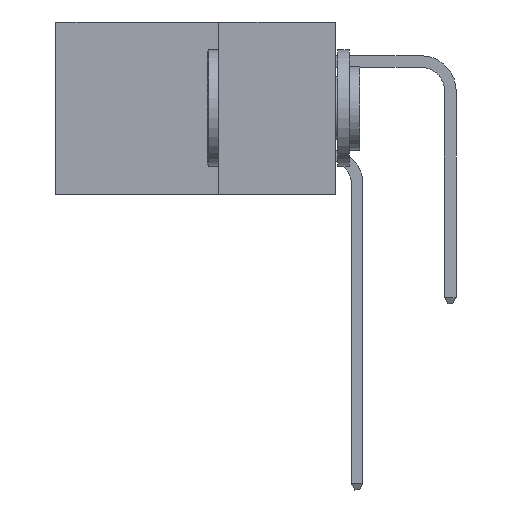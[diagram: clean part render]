
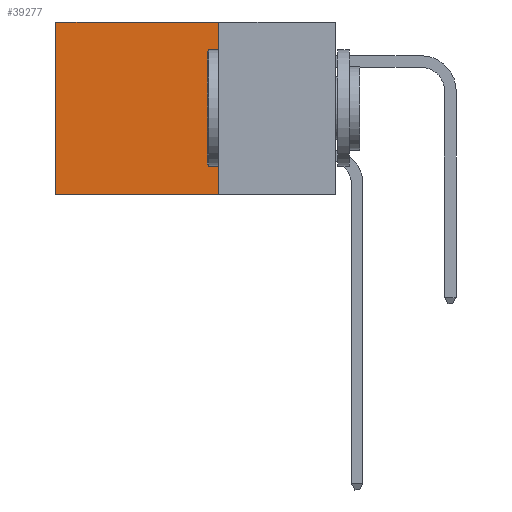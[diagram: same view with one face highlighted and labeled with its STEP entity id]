
A CAD part, left-side view. The second image highlights one B-rep face of the part: STEP entity #39277.
In plain terms, the highlighted planar face has unit normal (-1, 0, 0).
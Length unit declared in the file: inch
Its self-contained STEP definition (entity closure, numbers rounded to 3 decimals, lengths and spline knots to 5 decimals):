
#844 = VERTEX_POINT ( 'NONE', #34008 ) ;
#2474 = LINE ( 'NONE', #29731, #31496 ) ;
#5614 = VECTOR ( 'NONE', #31732, 39.37008 ) ;
#6262 = DIRECTION ( 'NONE',  ( 0., 0., -1. ) ) ;
#7840 = VECTOR ( 'NONE', #37528, 39.37008 ) ;
#9372 = DIRECTION ( 'NONE',  ( 0., 0., -1. ) ) ;
#11034 = VERTEX_POINT ( 'NONE', #16763 ) ;
#11585 = EDGE_CURVE ( 'NONE', #22320, #32104, #30597, .T. ) ;
#12231 = CARTESIAN_POINT ( 'NONE',  ( 0.2875, 0.25, -0.37 ) ) ;
#15916 = ORIENTED_EDGE ( 'NONE', *, *, #34098, .T. ) ;
#16762 = DIRECTION ( 'NONE',  ( 1., 0., 0. ) ) ;
#16763 = CARTESIAN_POINT ( 'NONE',  ( 0.2875, 0.25, 0. ) ) ;
#18892 = CARTESIAN_POINT ( 'NONE',  ( 0.2875, 0.25, -0.37 ) ) ;
#20705 = CARTESIAN_POINT ( 'NONE',  ( 0.2875, 0.25, 0. ) ) ;
#21686 = VECTOR ( 'NONE', #22266, 39.37008 ) ;
#22266 = DIRECTION ( 'NONE',  ( 0., 1., 0. ) ) ;
#22320 = VERTEX_POINT ( 'NONE', #12231 ) ;
#25436 = AXIS2_PLACEMENT_3D ( 'NONE', #36960, #16762, #6262 ) ;
#26860 = EDGE_CURVE ( 'NONE', #11034, #22320, #30504, .T. ) ;
#28300 = LINE ( 'NONE', #28796, #5614 ) ;
#28796 = CARTESIAN_POINT ( 'NONE',  ( 0.2875, 0.25, 0. ) ) ;
#29137 = FACE_OUTER_BOUND ( 'NONE', #35464, .T. ) ;
#29329 = ORIENTED_EDGE ( 'NONE', *, *, #26860, .F. ) ;
#29731 = CARTESIAN_POINT ( 'NONE',  ( 0.2875, 0.6, 0. ) ) ;
#30290 = ORIENTED_EDGE ( 'NONE', *, *, #34430, .T. ) ;
#30504 = LINE ( 'NONE', #20705, #7840 ) ;
#30597 = LINE ( 'NONE', #18892, #21686 ) ;
#31496 = VECTOR ( 'NONE', #9372, 39.37008 ) ;
#31732 = DIRECTION ( 'NONE',  ( 0., 1., 0. ) ) ;
#32104 = VERTEX_POINT ( 'NONE', #32429 ) ;
#32429 = CARTESIAN_POINT ( 'NONE',  ( 0.2875, 0.6, -0.37 ) ) ;
#33808 = PLANE ( 'NONE',  #25436 ) ;
#34008 = CARTESIAN_POINT ( 'NONE',  ( 0.2875, 0.6, 0. ) ) ;
#34098 = EDGE_CURVE ( 'NONE', #844, #32104, #2474, .T. ) ;
#34430 = EDGE_CURVE ( 'NONE', #11034, #844, #28300, .T. ) ;
#35464 = EDGE_LOOP ( 'NONE', ( #15916, #37296, #29329, #30290 ) ) ;
#36960 = CARTESIAN_POINT ( 'NONE',  ( 0.2875, 0.25, 0. ) ) ;
#37296 = ORIENTED_EDGE ( 'NONE', *, *, #11585, .F. ) ;
#37528 = DIRECTION ( 'NONE',  ( 0., 0., -1. ) ) ;
#39277 = ADVANCED_FACE ( 'NONE', ( #29137 ), #33808, .F. ) ;
